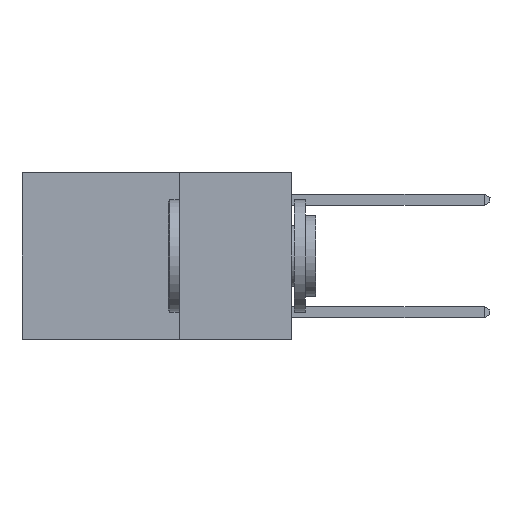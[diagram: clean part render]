
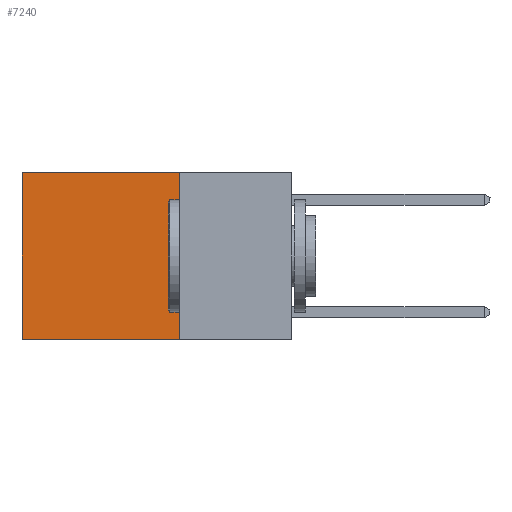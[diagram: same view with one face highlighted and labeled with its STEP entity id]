
A CAD part, left-side view. The second image highlights one B-rep face of the part: STEP entity #7240.
In plain terms, the highlighted planar face has unit normal (-1, 0, 0).
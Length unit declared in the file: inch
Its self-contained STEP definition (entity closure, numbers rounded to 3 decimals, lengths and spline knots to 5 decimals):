
#202 = LINE ( 'NONE', #5397, #8707 ) ;
#1820 = VECTOR ( 'NONE', #4723, 39.37008 ) ;
#1901 = ORIENTED_EDGE ( 'NONE', *, *, #11915, .T. ) ;
#1925 = PLANE ( 'NONE',  #6599 ) ;
#2408 = EDGE_CURVE ( 'NONE', #6982, #5592, #8306, .T. ) ;
#2877 = VECTOR ( 'NONE', #11920, 39.37008 ) ;
#2968 = FACE_OUTER_BOUND ( 'NONE', #5264, .T. ) ;
#3179 = VECTOR ( 'NONE', #9420, 39.37008 ) ;
#3270 = ORIENTED_EDGE ( 'NONE', *, *, #2408, .T. ) ;
#4663 = CARTESIAN_POINT ( 'NONE',  ( 0.2625, 0.6, -0.37 ) ) ;
#4723 = DIRECTION ( 'NONE',  ( 0., 1., 0. ) ) ;
#4739 = LINE ( 'NONE', #4867, #2877 ) ;
#4867 = CARTESIAN_POINT ( 'NONE',  ( 0.2625, 0.25, -0.37 ) ) ;
#5264 = EDGE_LOOP ( 'NONE', ( #3270, #7500, #11473, #1901 ) ) ;
#5397 = CARTESIAN_POINT ( 'NONE',  ( 0.2625, 0.25, 0. ) ) ;
#5592 = VERTEX_POINT ( 'NONE', #4663 ) ;
#5753 = CARTESIAN_POINT ( 'NONE',  ( 0.2625, 0.25, -0.37 ) ) ;
#5947 = CARTESIAN_POINT ( 'NONE',  ( 0.2625, 0.25, 0. ) ) ;
#6356 = CARTESIAN_POINT ( 'NONE',  ( 0.2625, 0.6, 0. ) ) ;
#6599 = AXIS2_PLACEMENT_3D ( 'NONE', #5947, #7005, #8953 ) ;
#6982 = VERTEX_POINT ( 'NONE', #11775 ) ;
#7005 = DIRECTION ( 'NONE',  ( 1., 0., 0. ) ) ;
#7240 = ADVANCED_FACE ( 'NONE', ( #2968 ), #1925, .F. ) ;
#7360 = DIRECTION ( 'NONE',  ( 0., 0., -1. ) ) ;
#7500 = ORIENTED_EDGE ( 'NONE', *, *, #12938, .F. ) ;
#7619 = LINE ( 'NONE', #11636, #1820 ) ;
#8306 = LINE ( 'NONE', #6356, #3179 ) ;
#8463 = VERTEX_POINT ( 'NONE', #9694 ) ;
#8707 = VECTOR ( 'NONE', #7360, 39.37008 ) ;
#8953 = DIRECTION ( 'NONE',  ( 0., 0., -1. ) ) ;
#9420 = DIRECTION ( 'NONE',  ( 0., 0., -1. ) ) ;
#9694 = CARTESIAN_POINT ( 'NONE',  ( 0.2625, 0.25, 0. ) ) ;
#10897 = EDGE_CURVE ( 'NONE', #8463, #11534, #202, .T. ) ;
#11473 = ORIENTED_EDGE ( 'NONE', *, *, #10897, .F. ) ;
#11534 = VERTEX_POINT ( 'NONE', #5753 ) ;
#11636 = CARTESIAN_POINT ( 'NONE',  ( 0.2625, 0.25, 0. ) ) ;
#11775 = CARTESIAN_POINT ( 'NONE',  ( 0.2625, 0.6, 0. ) ) ;
#11915 = EDGE_CURVE ( 'NONE', #8463, #6982, #7619, .T. ) ;
#11920 = DIRECTION ( 'NONE',  ( 0., 1., 0. ) ) ;
#12938 = EDGE_CURVE ( 'NONE', #11534, #5592, #4739, .T. ) ;
